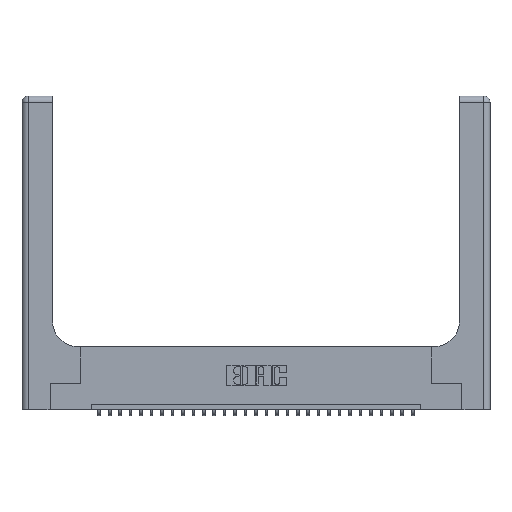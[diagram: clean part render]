
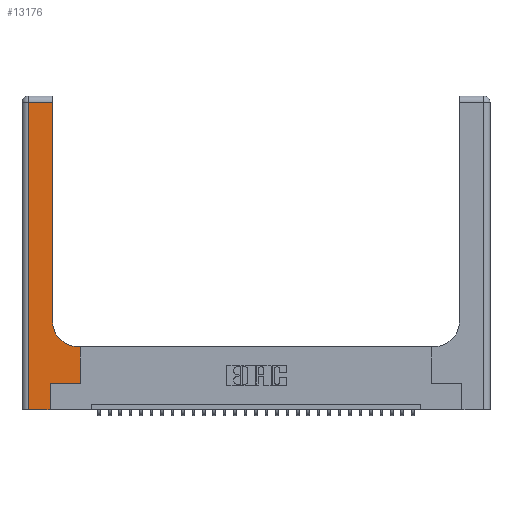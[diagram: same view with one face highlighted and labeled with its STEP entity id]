
A CAD part, top view. The second image highlights one B-rep face of the part: STEP entity #13176.
In plain terms, the highlighted planar face has unit normal (0, 0, 1).
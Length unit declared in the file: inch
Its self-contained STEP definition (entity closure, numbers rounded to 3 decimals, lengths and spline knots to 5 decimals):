
#57 = VECTOR ( 'NONE', #21739, 39.37008 ) ;
#841 = CARTESIAN_POINT ( 'NONE',  ( 0., 3., 0.37 ) ) ;
#858 = CARTESIAN_POINT ( 'NONE',  ( 0.2915, 0.6, 0.37 ) ) ;
#1129 = CARTESIAN_POINT ( 'NONE',  ( 0.5585, 0.25, 0.37 ) ) ;
#1456 = VERTEX_POINT ( 'NONE', #27363 ) ;
#1703 = ORIENTED_EDGE ( 'NONE', *, *, #29569, .T. ) ;
#1747 = CARTESIAN_POINT ( 'NONE',  ( 0.2915, 3., 0.37 ) ) ;
#2250 = VERTEX_POINT ( 'NONE', #5295 ) ;
#3106 = ORIENTED_EDGE ( 'NONE', *, *, #7747, .T. ) ;
#4761 = CARTESIAN_POINT ( 'NONE',  ( 0.5415, 0.6, 0.37 ) ) ;
#5029 = CARTESIAN_POINT ( 'NONE',  ( 0.5585, 0.6, 0.37 ) ) ;
#5295 = CARTESIAN_POINT ( 'NONE',  ( 0.06, 0., 0.37 ) ) ;
#5319 = DIRECTION ( 'NONE',  ( 0., 0., -1. ) ) ;
#5773 = ORIENTED_EDGE ( 'NONE', *, *, #7145, .T. ) ;
#6035 = VECTOR ( 'NONE', #8919, 39.37008 ) ;
#6050 = CARTESIAN_POINT ( 'NONE',  ( 0.269, 0., 0.37 ) ) ;
#6215 = LINE ( 'NONE', #7627, #57 ) ;
#6227 = VECTOR ( 'NONE', #7500, 39.37008 ) ;
#6245 = VERTEX_POINT ( 'NONE', #5029 ) ;
#6504 = VECTOR ( 'NONE', #19768, 39.37008 ) ;
#7145 = EDGE_CURVE ( 'NONE', #29317, #13595, #8796, .T. ) ;
#7230 = ORIENTED_EDGE ( 'NONE', *, *, #13997, .T. ) ;
#7237 = ORIENTED_EDGE ( 'NONE', *, *, #24035, .T. ) ;
#7500 = DIRECTION ( 'NONE',  ( 1., 0., 0. ) ) ;
#7627 = CARTESIAN_POINT ( 'NONE',  ( 0.269, 0.25, 0.37 ) ) ;
#7747 = EDGE_CURVE ( 'NONE', #13595, #23673, #6215, .T. ) ;
#7805 = CARTESIAN_POINT ( 'NONE',  ( 0.269, 0., 0.37 ) ) ;
#8498 = DIRECTION ( 'NONE',  ( 1., 0., 0. ) ) ;
#8736 = FACE_OUTER_BOUND ( 'NONE', #21823, .T. ) ;
#8796 = LINE ( 'NONE', #6050, #18941 ) ;
#8919 = DIRECTION ( 'NONE',  ( 0., -1., 0. ) ) ;
#9024 = DIRECTION ( 'NONE',  ( 0., 1., 0. ) ) ;
#10442 = LINE ( 'NONE', #1747, #21325 ) ;
#10484 = AXIS2_PLACEMENT_3D ( 'NONE', #841, #5319, #28861 ) ;
#10802 = CIRCLE ( 'NONE', #11457, 0.25 ) ;
#10849 = VERTEX_POINT ( 'NONE', #4761 ) ;
#11131 = CARTESIAN_POINT ( 'NONE',  ( 0.269, 0.25, 0.37 ) ) ;
#11457 = AXIS2_PLACEMENT_3D ( 'NONE', #29014, #29114, #8498 ) ;
#12526 = DIRECTION ( 'NONE',  ( 0., 1., 0. ) ) ;
#13176 = ADVANCED_FACE ( 'NONE', ( #8736 ), #21469, .F. ) ;
#13595 = VERTEX_POINT ( 'NONE', #11131 ) ;
#13945 = LINE ( 'NONE', #20307, #19383 ) ;
#13997 = EDGE_CURVE ( 'NONE', #10849, #25084, #10802, .T. ) ;
#14094 = ORIENTED_EDGE ( 'NONE', *, *, #26632, .T. ) ;
#14266 = DIRECTION ( 'NONE',  ( -1., 0., 0. ) ) ;
#14371 = EDGE_CURVE ( 'NONE', #25557, #1456, #18395, .T. ) ;
#15666 = CARTESIAN_POINT ( 'NONE',  ( 0.2915, 0.85, 0.37 ) ) ;
#18395 = LINE ( 'NONE', #21464, #19502 ) ;
#18941 = VECTOR ( 'NONE', #12526, 39.37008 ) ;
#19383 = VECTOR ( 'NONE', #9024, 39.37008 ) ;
#19502 = VECTOR ( 'NONE', #14266, 39.37008 ) ;
#19685 = EDGE_CURVE ( 'NONE', #6245, #10849, #25032, .T. ) ;
#19768 = DIRECTION ( 'NONE',  ( -1., 0., 0. ) ) ;
#19928 = CARTESIAN_POINT ( 'NONE',  ( 0.2915, 2.94, 0.37 ) ) ;
#20302 = ORIENTED_EDGE ( 'NONE', *, *, #14371, .T. ) ;
#20307 = CARTESIAN_POINT ( 'NONE',  ( 0.5585, 0.25, 0.37 ) ) ;
#21213 = EDGE_CURVE ( 'NONE', #1456, #2250, #24550, .T. ) ;
#21325 = VECTOR ( 'NONE', #27422, 39.37008 ) ;
#21464 = CARTESIAN_POINT ( 'NONE',  ( 0., 2.94, 0.37 ) ) ;
#21469 = PLANE ( 'NONE',  #10484 ) ;
#21739 = DIRECTION ( 'NONE',  ( 1., 0., 0. ) ) ;
#21823 = EDGE_LOOP ( 'NONE', ( #14094, #20302, #23866, #7237, #5773, #3106, #1703, #25214, #7230 ) ) ;
#23059 = CARTESIAN_POINT ( 'NONE',  ( 0., 0., 0.37 ) ) ;
#23673 = VERTEX_POINT ( 'NONE', #1129 ) ;
#23866 = ORIENTED_EDGE ( 'NONE', *, *, #21213, .T. ) ;
#24035 = EDGE_CURVE ( 'NONE', #2250, #29317, #26927, .T. ) ;
#24550 = LINE ( 'NONE', #24940, #6035 ) ;
#24940 = CARTESIAN_POINT ( 'NONE',  ( 0.06, 3., 0.37 ) ) ;
#25032 = LINE ( 'NONE', #858, #6504 ) ;
#25084 = VERTEX_POINT ( 'NONE', #15666 ) ;
#25214 = ORIENTED_EDGE ( 'NONE', *, *, #19685, .T. ) ;
#25557 = VERTEX_POINT ( 'NONE', #19928 ) ;
#26632 = EDGE_CURVE ( 'NONE', #25084, #25557, #10442, .T. ) ;
#26927 = LINE ( 'NONE', #23059, #6227 ) ;
#27363 = CARTESIAN_POINT ( 'NONE',  ( 0.06, 2.94, 0.37 ) ) ;
#27422 = DIRECTION ( 'NONE',  ( 0., 1., 0. ) ) ;
#28861 = DIRECTION ( 'NONE',  ( -1., 0., 0. ) ) ;
#29014 = CARTESIAN_POINT ( 'NONE',  ( 0.5415, 0.85, 0.37 ) ) ;
#29114 = DIRECTION ( 'NONE',  ( 0., 0., -1. ) ) ;
#29317 = VERTEX_POINT ( 'NONE', #7805 ) ;
#29569 = EDGE_CURVE ( 'NONE', #23673, #6245, #13945, .T. ) ;
